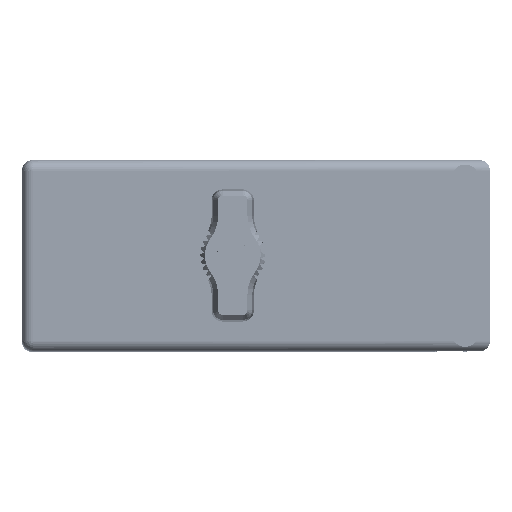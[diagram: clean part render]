
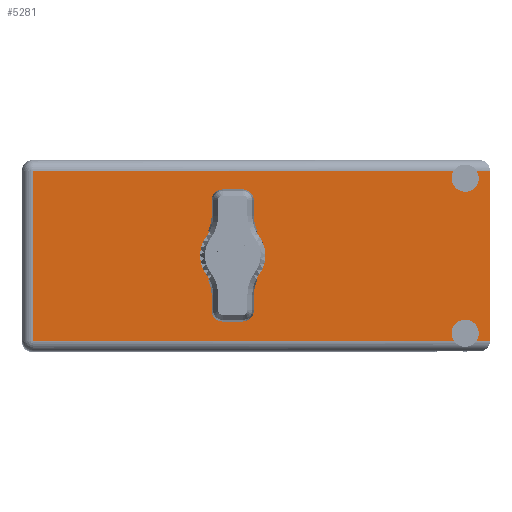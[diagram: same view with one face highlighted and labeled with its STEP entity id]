
A CAD part, top view. The second image highlights one B-rep face of the part: STEP entity #5281.
In plain terms, the highlighted face is planar.
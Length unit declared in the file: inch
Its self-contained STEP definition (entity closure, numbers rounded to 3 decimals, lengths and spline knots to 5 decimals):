
#1169 = DIRECTION ( 'NONE',  ( -1., 0., 0. ) ) ;
#2812 = EDGE_CURVE ( 'NONE', #54615, #93657, #48517, .T. ) ;
#4333 = ORIENTED_EDGE ( 'NONE', *, *, #51979, .F. ) ;
#5110 = DIRECTION ( 'NONE',  ( 0., 0., 1. ) ) ;
#5281 = ADVANCED_FACE ( 'NONE', ( #82164, #18359 ), #27649, .T. ) ;
#5365 = CARTESIAN_POINT ( 'NONE',  ( 0.07, 1.775, -0.07 ) ) ;
#6596 = EDGE_CURVE ( 'NONE', #92429, #61480, #77691, .T. ) ;
#7557 = ORIENTED_EDGE ( 'NONE', *, *, #36712, .T. ) ;
#9582 = AXIS2_PLACEMENT_3D ( 'NONE', #50310, #59254, #89722 ) ;
#11022 = DIRECTION ( 'NONE',  ( 0., 0., 1. ) ) ;
#12483 = CARTESIAN_POINT ( 'NONE',  ( 1.359, 1.775, -0.617 ) ) ;
#12553 = CARTESIAN_POINT ( 'NONE',  ( 0., 1.775, -1.164 ) ) ;
#12579 = VECTOR ( 'NONE', #93528, 39.37008 ) ;
#13643 = DIRECTION ( 'NONE',  ( 0., 0., 1. ) ) ;
#14481 = DIRECTION ( 'NONE',  ( 0., 0., 1. ) ) ;
#14676 = EDGE_CURVE ( 'NONE', #15581, #48847, #46918, .T. ) ;
#14735 = CARTESIAN_POINT ( 'NONE',  ( 2.858, 1.775, -1.117 ) ) ;
#15042 = CARTESIAN_POINT ( 'NONE',  ( 2.78419, 1.775, -0.07 ) ) ;
#15581 = VERTEX_POINT ( 'NONE', #66438 ) ;
#15742 = DIRECTION ( 'NONE',  ( 0., 0., 1. ) ) ;
#18359 = FACE_OUTER_BOUND ( 'NONE', #21626, .T. ) ;
#18585 = ORIENTED_EDGE ( 'NONE', *, *, #59861, .F. ) ;
#20036 = CARTESIAN_POINT ( 'NONE',  ( 0.07, 1.775, -1.234 ) ) ;
#20560 = CARTESIAN_POINT ( 'NONE',  ( 3.018, 1.775, -0.07 ) ) ;
#21135 = VERTEX_POINT ( 'NONE', #71916 ) ;
#21413 = AXIS2_PLACEMENT_3D ( 'NONE', #49104, #72079, #88049 ) ;
#21626 = EDGE_LOOP ( 'NONE', ( #90131, #48546, #4333, #93060, #49159, #57632, #81301, #43221, #96405, #7557 ) ) ;
#22395 = CARTESIAN_POINT ( 'NONE',  ( 3.018, 1.775, -0.07 ) ) ;
#23845 = AXIS2_PLACEMENT_3D ( 'NONE', #12483, #41060, #11022 ) ;
#26152 = CIRCLE ( 'NONE', #37359, 0.0875 ) ;
#26226 = DIRECTION ( 'NONE',  ( 0., 0., 1. ) ) ;
#27067 = DIRECTION ( 'NONE',  ( 1., 0., 0. ) ) ;
#27649 = PLANE ( 'NONE',  #32701 ) ;
#30549 = VERTEX_POINT ( 'NONE', #73896 ) ;
#30984 = CARTESIAN_POINT ( 'NONE',  ( 3.018, 1.775, 0. ) ) ;
#31306 = AXIS2_PLACEMENT_3D ( 'NONE', #80171, #43171, #5110 ) ;
#32503 = LINE ( 'NONE', #63053, #12579 ) ;
#32701 = AXIS2_PLACEMENT_3D ( 'NONE', #81680, #58204, #13643 ) ;
#33362 = CARTESIAN_POINT ( 'NONE',  ( 1.359, 1.775, -0.492 ) ) ;
#34753 = VERTEX_POINT ( 'NONE', #54714 ) ;
#36712 = EDGE_CURVE ( 'NONE', #34753, #40879, #89515, .T. ) ;
#37359 = AXIS2_PLACEMENT_3D ( 'NONE', #14735, #68778, #15742 ) ;
#37666 = VERTEX_POINT ( 'NONE', #74608 ) ;
#38778 = CARTESIAN_POINT ( 'NONE',  ( 1.359, 1.775, -0.617 ) ) ;
#39180 = CARTESIAN_POINT ( 'NONE',  ( 0., 1.775, -1.164 ) ) ;
#40879 = VERTEX_POINT ( 'NONE', #5365 ) ;
#41060 = DIRECTION ( 'NONE',  ( 0., 1., 0. ) ) ;
#42126 = CARTESIAN_POINT ( 'NONE',  ( 3.018, 1.775, -1.164 ) ) ;
#42603 = LINE ( 'NONE', #22395, #92729 ) ;
#43003 = CIRCLE ( 'NONE', #23845, 0.125 ) ;
#43171 = DIRECTION ( 'NONE',  ( 0., 1., 0. ) ) ;
#43221 = ORIENTED_EDGE ( 'NONE', *, *, #78342, .F. ) ;
#46918 = CIRCLE ( 'NONE', #31306, 0.0875 ) ;
#47192 = CARTESIAN_POINT ( 'NONE',  ( 2.93181, 1.775, -1.164 ) ) ;
#47295 = AXIS2_PLACEMENT_3D ( 'NONE', #38778, #69299, #26226 ) ;
#48517 = LINE ( 'NONE', #30984, #54944 ) ;
#48546 = ORIENTED_EDGE ( 'NONE', *, *, #86962, .F. ) ;
#48847 = VERTEX_POINT ( 'NONE', #47192 ) ;
#49104 = CARTESIAN_POINT ( 'NONE',  ( 2.858, 1.775, -0.117 ) ) ;
#49159 = ORIENTED_EDGE ( 'NONE', *, *, #2812, .F. ) ;
#50310 = CARTESIAN_POINT ( 'NONE',  ( 2.858, 1.775, -0.117 ) ) ;
#51979 = EDGE_CURVE ( 'NONE', #21135, #30549, #66152, .T. ) ;
#54172 = VECTOR ( 'NONE', #80587, 39.37008 ) ;
#54615 = VERTEX_POINT ( 'NONE', #42126 ) ;
#54714 = CARTESIAN_POINT ( 'NONE',  ( 0.07, 1.775, -1.164 ) ) ;
#54944 = VECTOR ( 'NONE', #92995, 39.37008 ) ;
#57632 = ORIENTED_EDGE ( 'NONE', *, *, #62907, .T. ) ;
#58204 = DIRECTION ( 'NONE',  ( 0., 1., 0. ) ) ;
#59254 = DIRECTION ( 'NONE',  ( 0., 1., 0. ) ) ;
#59861 = EDGE_CURVE ( 'NONE', #61480, #92429, #43003, .T. ) ;
#61254 = EDGE_CURVE ( 'NONE', #40879, #91605, #42603, .T. ) ;
#61480 = VERTEX_POINT ( 'NONE', #33362 ) ;
#62192 = LINE ( 'NONE', #39180, #81066 ) ;
#62907 = EDGE_CURVE ( 'NONE', #54615, #48847, #62192, .T. ) ;
#63053 = CARTESIAN_POINT ( 'NONE',  ( 3.018, 1.775, -0.07 ) ) ;
#64730 = EDGE_CURVE ( 'NONE', #37666, #34753, #81084, .T. ) ;
#66152 = CIRCLE ( 'NONE', #21413, 0.0875 ) ;
#66409 = EDGE_CURVE ( 'NONE', #21135, #93657, #32503, .T. ) ;
#66438 = CARTESIAN_POINT ( 'NONE',  ( 2.858, 1.775, -1.0295 ) ) ;
#67792 = CARTESIAN_POINT ( 'NONE',  ( 1.359, 1.775, -0.742 ) ) ;
#68778 = DIRECTION ( 'NONE',  ( 0., 1., 0. ) ) ;
#69299 = DIRECTION ( 'NONE',  ( 0., 1., 0. ) ) ;
#71916 = CARTESIAN_POINT ( 'NONE',  ( 2.93181, 1.775, -0.07 ) ) ;
#72079 = DIRECTION ( 'NONE',  ( 0., 1., 0. ) ) ;
#73896 = CARTESIAN_POINT ( 'NONE',  ( 2.858, 1.775, -0.2045 ) ) ;
#74608 = CARTESIAN_POINT ( 'NONE',  ( 2.78419, 1.775, -1.164 ) ) ;
#75027 = CIRCLE ( 'NONE', #9582, 0.0875 ) ;
#77691 = CIRCLE ( 'NONE', #47295, 0.125 ) ;
#78342 = EDGE_CURVE ( 'NONE', #37666, #15581, #26152, .T. ) ;
#80171 = CARTESIAN_POINT ( 'NONE',  ( 2.858, 1.775, -1.117 ) ) ;
#80587 = DIRECTION ( 'NONE',  ( -1., 0., 0. ) ) ;
#81066 = VECTOR ( 'NONE', #1169, 39.37008 ) ;
#81084 = LINE ( 'NONE', #12553, #54172 ) ;
#81301 = ORIENTED_EDGE ( 'NONE', *, *, #14676, .F. ) ;
#81680 = CARTESIAN_POINT ( 'NONE',  ( 0., 1.775, -1.234 ) ) ;
#82164 = FACE_BOUND ( 'NONE', #95422, .T. ) ;
#86962 = EDGE_CURVE ( 'NONE', #30549, #91605, #75027, .T. ) ;
#87188 = VECTOR ( 'NONE', #14481, 39.37008 ) ;
#88049 = DIRECTION ( 'NONE',  ( 0., 0., 1. ) ) ;
#89515 = LINE ( 'NONE', #20036, #87188 ) ;
#89722 = DIRECTION ( 'NONE',  ( 0., 0., 1. ) ) ;
#90131 = ORIENTED_EDGE ( 'NONE', *, *, #61254, .T. ) ;
#91605 = VERTEX_POINT ( 'NONE', #15042 ) ;
#92429 = VERTEX_POINT ( 'NONE', #67792 ) ;
#92729 = VECTOR ( 'NONE', #27067, 39.37008 ) ;
#92995 = DIRECTION ( 'NONE',  ( 0., 0., 1. ) ) ;
#93060 = ORIENTED_EDGE ( 'NONE', *, *, #66409, .T. ) ;
#93528 = DIRECTION ( 'NONE',  ( 1., 0., 0. ) ) ;
#93657 = VERTEX_POINT ( 'NONE', #20560 ) ;
#95422 = EDGE_LOOP ( 'NONE', ( #18585, #98790 ) ) ;
#96405 = ORIENTED_EDGE ( 'NONE', *, *, #64730, .T. ) ;
#98790 = ORIENTED_EDGE ( 'NONE', *, *, #6596, .F. ) ;
